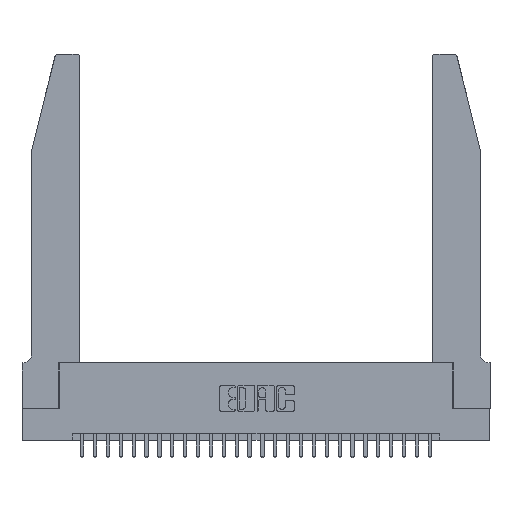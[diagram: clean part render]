
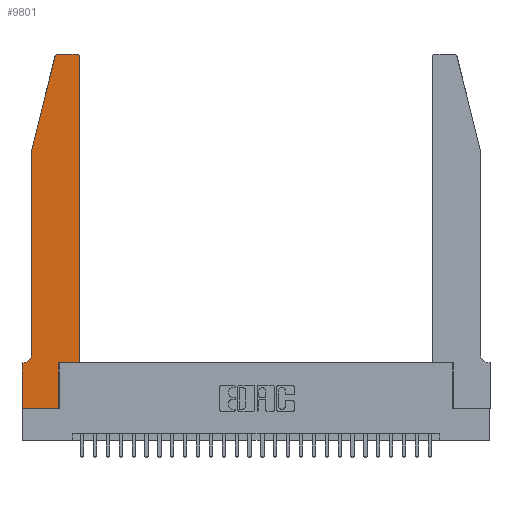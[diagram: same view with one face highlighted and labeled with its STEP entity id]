
A CAD part, top view. The second image highlights one B-rep face of the part: STEP entity #9801.
In plain terms, the highlighted planar face has unit normal (0, 0, 1).
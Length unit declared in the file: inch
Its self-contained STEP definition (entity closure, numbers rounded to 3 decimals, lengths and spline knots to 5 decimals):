
#241 = CARTESIAN_POINT ( 'NONE',  ( 0.2865, 0.35, 0.37 ) ) ;
#579 = DIRECTION ( 'NONE',  ( 0., -1., 0. ) ) ;
#912 = DIRECTION ( 'NONE',  ( 0., -1., 0. ) ) ;
#1289 = VERTEX_POINT ( 'NONE', #28077 ) ;
#1427 = CARTESIAN_POINT ( 'NONE',  ( 0.2865, 0., 0.37 ) ) ;
#1472 = VERTEX_POINT ( 'NONE', #16917 ) ;
#1688 = DIRECTION ( 'NONE',  ( 1., 0., 0. ) ) ;
#1871 = DIRECTION ( 'NONE',  ( 0., 0., 1. ) ) ;
#2201 = VERTEX_POINT ( 'NONE', #13247 ) ;
#2378 = ORIENTED_EDGE ( 'NONE', *, *, #19692, .T. ) ;
#3819 = DIRECTION ( 'NONE',  ( 1., 0., 0. ) ) ;
#3893 = EDGE_CURVE ( 'NONE', #9358, #1472, #25101, .T. ) ;
#3902 = VERTEX_POINT ( 'NONE', #12734 ) ;
#4038 = CARTESIAN_POINT ( 'NONE',  ( 0.0755, 0.42, 0.37 ) ) ;
#4608 = DIRECTION ( 'NONE',  ( -1., 0., 0. ) ) ;
#4653 = VECTOR ( 'NONE', #26074, 39.37008 ) ;
#4726 = VECTOR ( 'NONE', #21197, 39.37008 ) ;
#4962 = CARTESIAN_POINT ( 'NONE',  ( 0.4505, 0.35, 0.37 ) ) ;
#5230 = ORIENTED_EDGE ( 'NONE', *, *, #22885, .T. ) ;
#5604 = ORIENTED_EDGE ( 'NONE', *, *, #25147, .T. ) ;
#5770 = EDGE_CURVE ( 'NONE', #28530, #28079, #15698, .T. ) ;
#5789 = ORIENTED_EDGE ( 'NONE', *, *, #14219, .T. ) ;
#6067 = LINE ( 'NONE', #14855, #4653 ) ;
#6113 = CARTESIAN_POINT ( 'NONE',  ( 0.4205, 2.72, 0.37 ) ) ;
#6128 = AXIS2_PLACEMENT_3D ( 'NONE', #6113, #19183, #14820 ) ;
#6139 = DIRECTION ( 'NONE',  ( 0., 1., 0. ) ) ;
#7134 = CARTESIAN_POINT ( 'NONE',  ( 0.0755, 2., 0.37 ) ) ;
#7474 = ORIENTED_EDGE ( 'NONE', *, *, #5770, .T. ) ;
#7651 = CIRCLE ( 'NONE', #26270, 0.07 ) ;
#7981 = CARTESIAN_POINT ( 'NONE',  ( 0.4505, 2.72, 0.37 ) ) ;
#8137 = EDGE_CURVE ( 'NONE', #8917, #18535, #8816, .T. ) ;
#8402 = VECTOR ( 'NONE', #579, 39.37008 ) ;
#8587 = CARTESIAN_POINT ( 'NONE',  ( 0.4505, 0.35, 0.37 ) ) ;
#8816 = LINE ( 'NONE', #25204, #25748 ) ;
#8917 = VERTEX_POINT ( 'NONE', #7134 ) ;
#9092 = ORIENTED_EDGE ( 'NONE', *, *, #26569, .T. ) ;
#9145 = EDGE_CURVE ( 'NONE', #3902, #23604, #15625, .T. ) ;
#9171 = DIRECTION ( 'NONE',  ( 1., 0., 0. ) ) ;
#9280 = VECTOR ( 'NONE', #23283, 39.37008 ) ;
#9358 = VERTEX_POINT ( 'NONE', #7981 ) ;
#9801 = ADVANCED_FACE ( 'NONE', ( #15257 ), #16988, .T. ) ;
#9978 = CARTESIAN_POINT ( 'NONE',  ( 0., 0., 0.37 ) ) ;
#9986 = LINE ( 'NONE', #21681, #4726 ) ;
#10370 = VERTEX_POINT ( 'NONE', #24969 ) ;
#10728 = DIRECTION ( 'NONE',  ( -0.239, -0.971, 0. ) ) ;
#10938 = CARTESIAN_POINT ( 'NONE',  ( 0., 0., 0.37 ) ) ;
#11096 = ORIENTED_EDGE ( 'NONE', *, *, #12402, .T. ) ;
#11098 = CARTESIAN_POINT ( 'NONE',  ( 0.0755, 2., 0.37 ) ) ;
#11573 = AXIS2_PLACEMENT_3D ( 'NONE', #21813, #1871, #1688 ) ;
#11875 = VECTOR ( 'NONE', #9171, 39.37008 ) ;
#12043 = ORIENTED_EDGE ( 'NONE', *, *, #16017, .T. ) ;
#12113 = VECTOR ( 'NONE', #10728, 39.37008 ) ;
#12203 = ORIENTED_EDGE ( 'NONE', *, *, #19175, .T. ) ;
#12402 = EDGE_CURVE ( 'NONE', #24092, #9358, #21417, .T. ) ;
#12734 = CARTESIAN_POINT ( 'NONE',  ( 0., 0.35, 0.37 ) ) ;
#13247 = CARTESIAN_POINT ( 'NONE',  ( 0.284, 2.75, 0.37 ) ) ;
#13892 = CARTESIAN_POINT ( 'NONE',  ( 0.4505, 0.35, 0.37 ) ) ;
#14063 = VECTOR ( 'NONE', #20588, 39.37008 ) ;
#14219 = EDGE_CURVE ( 'NONE', #28079, #24092, #17490, .T. ) ;
#14549 = ORIENTED_EDGE ( 'NONE', *, *, #9145, .T. ) ;
#14820 = DIRECTION ( 'NONE',  ( 1., 0., 0. ) ) ;
#14855 = CARTESIAN_POINT ( 'NONE',  ( 0.2605, 2.75, 0.37 ) ) ;
#15257 = FACE_OUTER_BOUND ( 'NONE', #21357, .T. ) ;
#15625 = LINE ( 'NONE', #9978, #8402 ) ;
#15698 = LINE ( 'NONE', #28386, #25054 ) ;
#15999 = CARTESIAN_POINT ( 'NONE',  ( 0., 0., 0.37 ) ) ;
#16017 = EDGE_CURVE ( 'NONE', #23604, #28530, #17734, .T. ) ;
#16917 = CARTESIAN_POINT ( 'NONE',  ( 0.4205, 2.75, 0.37 ) ) ;
#16988 = PLANE ( 'NONE',  #19773 ) ;
#17427 = DIRECTION ( 'NONE',  ( 0., 0., -1. ) ) ;
#17490 = LINE ( 'NONE', #4962, #14063 ) ;
#17734 = LINE ( 'NONE', #15999, #11875 ) ;
#17927 = LINE ( 'NONE', #11098, #12113 ) ;
#18535 = VERTEX_POINT ( 'NONE', #4038 ) ;
#19175 = EDGE_CURVE ( 'NONE', #1289, #8917, #17927, .T. ) ;
#19183 = DIRECTION ( 'NONE',  ( 0., 0., 1. ) ) ;
#19692 = EDGE_CURVE ( 'NONE', #2201, #1289, #22775, .T. ) ;
#19773 = AXIS2_PLACEMENT_3D ( 'NONE', #21670, #23912, #3819 ) ;
#20588 = DIRECTION ( 'NONE',  ( 1., 0., 0. ) ) ;
#21197 = DIRECTION ( 'NONE',  ( -1., 0., 0. ) ) ;
#21357 = EDGE_LOOP ( 'NONE', ( #9092, #2378, #12203, #21736, #5230, #5604, #14549, #12043, #7474, #5789, #11096, #27789 ) ) ;
#21417 = LINE ( 'NONE', #13892, #9280 ) ;
#21670 = CARTESIAN_POINT ( 'NONE',  ( 0., 0.35, 0.37 ) ) ;
#21681 = CARTESIAN_POINT ( 'NONE',  ( 0.0755, 0.35, 0.37 ) ) ;
#21736 = ORIENTED_EDGE ( 'NONE', *, *, #8137, .T. ) ;
#21813 = CARTESIAN_POINT ( 'NONE',  ( 0.284, 2.72, 0.37 ) ) ;
#22775 = CIRCLE ( 'NONE', #11573, 0.03 ) ;
#22885 = EDGE_CURVE ( 'NONE', #18535, #10370, #7651, .T. ) ;
#23283 = DIRECTION ( 'NONE',  ( 0., 1., 0. ) ) ;
#23604 = VERTEX_POINT ( 'NONE', #10938 ) ;
#23912 = DIRECTION ( 'NONE',  ( 0., 0., 1. ) ) ;
#24092 = VERTEX_POINT ( 'NONE', #8587 ) ;
#24969 = CARTESIAN_POINT ( 'NONE',  ( 0.0055, 0.35, 0.37 ) ) ;
#25054 = VECTOR ( 'NONE', #6139, 39.37008 ) ;
#25101 = CIRCLE ( 'NONE', #6128, 0.03 ) ;
#25147 = EDGE_CURVE ( 'NONE', #10370, #3902, #9986, .T. ) ;
#25204 = CARTESIAN_POINT ( 'NONE',  ( 0.0755, 2., 0.37 ) ) ;
#25748 = VECTOR ( 'NONE', #912, 39.37008 ) ;
#26074 = DIRECTION ( 'NONE',  ( -1., 0., 0. ) ) ;
#26270 = AXIS2_PLACEMENT_3D ( 'NONE', #27988, #17427, #4608 ) ;
#26569 = EDGE_CURVE ( 'NONE', #1472, #2201, #6067, .T. ) ;
#27789 = ORIENTED_EDGE ( 'NONE', *, *, #3893, .T. ) ;
#27988 = CARTESIAN_POINT ( 'NONE',  ( 0.0055, 0.42, 0.37 ) ) ;
#28077 = CARTESIAN_POINT ( 'NONE',  ( 0.25487, 2.72718, 0.37 ) ) ;
#28079 = VERTEX_POINT ( 'NONE', #241 ) ;
#28386 = CARTESIAN_POINT ( 'NONE',  ( 0.2865, 0.35, 0.37 ) ) ;
#28530 = VERTEX_POINT ( 'NONE', #1427 ) ;
